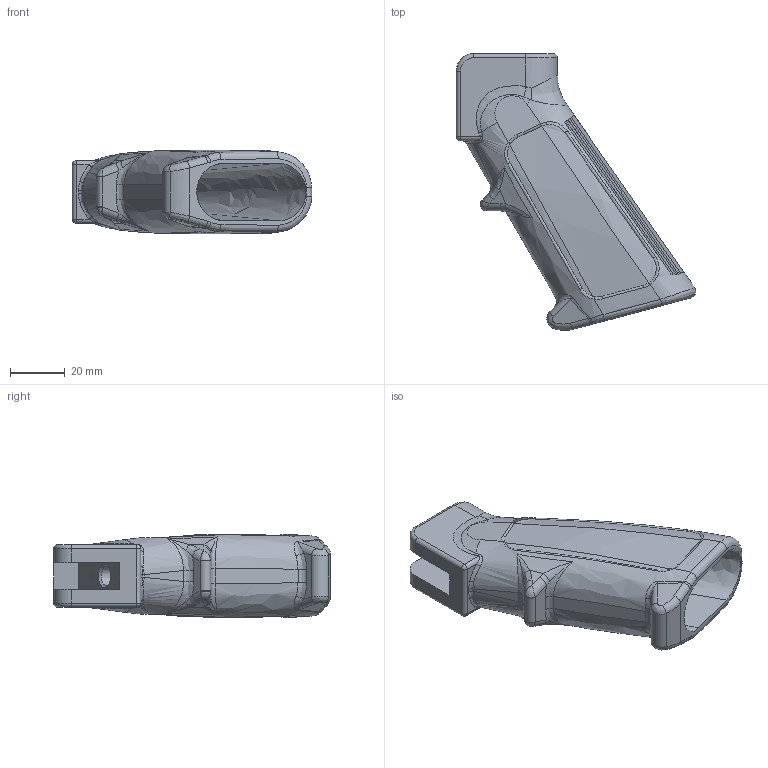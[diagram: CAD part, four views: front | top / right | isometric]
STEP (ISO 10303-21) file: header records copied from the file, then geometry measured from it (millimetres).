
FILE_DESCRIPTION(/* description */ (''),/* implementation_level */ '2;1');
FILE_NAME(/* name */ 'AR Pistol Grip.stp',/* time_stamp */ '2020-07-16T15:40:41-04:00',/* author */ ('flyin'),/* organization */ (''),/* preprocessor_version */ 'ST-DEVELOPER v17',/* originating_system */ 'Autodesk Inventor 2019',/* authorisation */ '');
FILE_SCHEMA (('AUTOMOTIVE_DESIGN { 1 0 10303 214 3 1 1 }'));
Length unit declared in the file: millimetre
Products named in the file (1): AR Pistol Grip
Bounding box: 87.27 x 100.87 x 30.58 mm (x, y, z)
Volume: 61722.9 mm3; surface area: 24125.4 mm2
Topology: 1 solids, 1 shells, 217 faces, 556 edges, 334 vertices
Faces by surface type: bspline 102, plane 79, cylinder 29, torus 3, cone 2, sphere 2
Full cylindrical faces by diameter (mm): 3.962 x1, 7.142 x1
Entity records: 10680 total; most frequent: CARTESIAN_POINT 5904, ORIENTED_EDGE 1086, DIRECTION 737, EDGE_CURVE 543, VERTEX_POINT 334, AXIS2_PLACEMENT_3D 263, EDGE_LOOP 225, FACE_OUTER_BOUND 217
